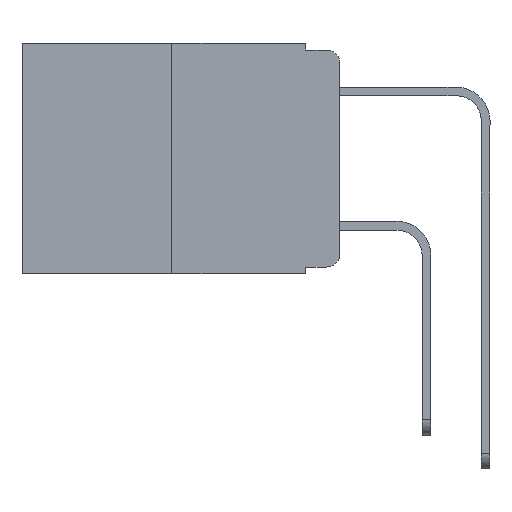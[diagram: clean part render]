
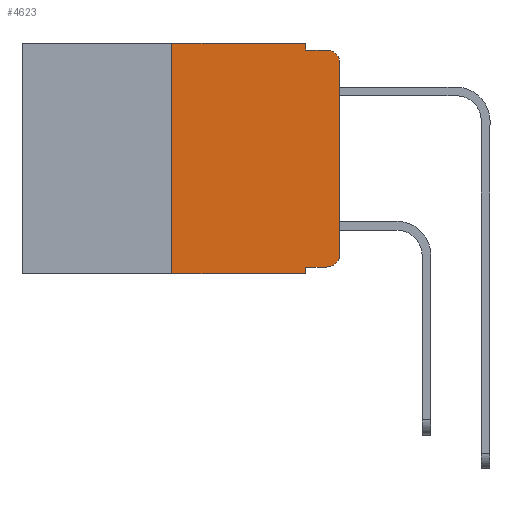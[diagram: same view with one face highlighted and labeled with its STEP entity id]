
A CAD part, left-side view. The second image highlights one B-rep face of the part: STEP entity #4623.
In plain terms, the highlighted planar face has unit normal (-1, 0, 0).
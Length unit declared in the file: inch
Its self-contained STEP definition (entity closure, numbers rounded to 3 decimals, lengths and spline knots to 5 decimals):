
#104 = VECTOR ( 'NONE', #4649, 39.37008 ) ;
#721 = ORIENTED_EDGE ( 'NONE', *, *, #9399, .F. ) ;
#742 = VERTEX_POINT ( 'NONE', #12933 ) ;
#1027 = AXIS2_PLACEMENT_3D ( 'NONE', #5376, #12724, #6508 ) ;
#1413 = CIRCLE ( 'NONE', #1027, 0.02 ) ;
#1497 = CARTESIAN_POINT ( 'NONE',  ( 0., 0.473, -0.343 ) ) ;
#1637 = DIRECTION ( 'NONE',  ( 0., -1., 0. ) ) ;
#1709 = CARTESIAN_POINT ( 'NONE',  ( 0., 0.02, -0.01 ) ) ;
#1729 = EDGE_LOOP ( 'NONE', ( #3747, #9186, #721, #8154, #5910, #5442, #3701, #11377, #7522, #10274 ) ) ;
#2589 = DIRECTION ( 'NONE',  ( 0., -1., 0. ) ) ;
#2990 = CARTESIAN_POINT ( 'NONE',  ( 0., 0.051, -0.333 ) ) ;
#2999 = LINE ( 'NONE', #11617, #8908 ) ;
#3168 = CARTESIAN_POINT ( 'NONE',  ( 0., 0.051, -0.343 ) ) ;
#3259 = VERTEX_POINT ( 'NONE', #11112 ) ;
#3571 = AXIS2_PLACEMENT_3D ( 'NONE', #6929, #10416, #8793 ) ;
#3701 = ORIENTED_EDGE ( 'NONE', *, *, #12202, .T. ) ;
#3729 = VERTEX_POINT ( 'NONE', #7700 ) ;
#3747 = ORIENTED_EDGE ( 'NONE', *, *, #4764, .T. ) ;
#3882 = CARTESIAN_POINT ( 'NONE',  ( 0., 0.473, 0. ) ) ;
#3914 = VECTOR ( 'NONE', #7093, 39.37008 ) ;
#4100 = EDGE_CURVE ( 'NONE', #3259, #742, #5727, .T. ) ;
#4226 = AXIS2_PLACEMENT_3D ( 'NONE', #11518, #11501, #5361 ) ;
#4256 = LINE ( 'NONE', #11847, #9707 ) ;
#4446 = VERTEX_POINT ( 'NONE', #7901 ) ;
#4544 = VERTEX_POINT ( 'NONE', #11835 ) ;
#4623 = ADVANCED_FACE ( 'NONE', ( #13670 ), #11587, .F. ) ;
#4649 = DIRECTION ( 'NONE',  ( 0., 0., -1. ) ) ;
#4717 = CARTESIAN_POINT ( 'NONE',  ( 0., 0.051, 0. ) ) ;
#4764 = EDGE_CURVE ( 'NONE', #4925, #4544, #12426, .T. ) ;
#4925 = VERTEX_POINT ( 'NONE', #12439 ) ;
#4958 = CIRCLE ( 'NONE', #3571, 0.02 ) ;
#5225 = DIRECTION ( 'NONE',  ( 0., 0., 1. ) ) ;
#5226 = DIRECTION ( 'NONE',  ( 0., 0., -1. ) ) ;
#5293 = LINE ( 'NONE', #7303, #8558 ) ;
#5361 = DIRECTION ( 'NONE',  ( 0., 0., -1. ) ) ;
#5376 = CARTESIAN_POINT ( 'NONE',  ( 0., 0.02, -0.313 ) ) ;
#5442 = ORIENTED_EDGE ( 'NONE', *, *, #9264, .F. ) ;
#5491 = VECTOR ( 'NONE', #1637, 39.37008 ) ;
#5637 = EDGE_CURVE ( 'NONE', #6915, #3729, #9873, .T. ) ;
#5727 = LINE ( 'NONE', #4717, #104 ) ;
#5807 = LINE ( 'NONE', #1497, #11384 ) ;
#5910 = ORIENTED_EDGE ( 'NONE', *, *, #9941, .F. ) ;
#5978 = VERTEX_POINT ( 'NONE', #1709 ) ;
#6288 = EDGE_CURVE ( 'NONE', #4544, #5978, #4958, .T. ) ;
#6392 = VERTEX_POINT ( 'NONE', #3168 ) ;
#6508 = DIRECTION ( 'NONE',  ( 0., 0., -1. ) ) ;
#6689 = EDGE_CURVE ( 'NONE', #6915, #6392, #5293, .T. ) ;
#6915 = VERTEX_POINT ( 'NONE', #2990 ) ;
#6929 = CARTESIAN_POINT ( 'NONE',  ( 0., 0.02, -0.03 ) ) ;
#6930 = CARTESIAN_POINT ( 'NONE',  ( 0., 0., 0. ) ) ;
#7093 = DIRECTION ( 'NONE',  ( 0., 0., 1. ) ) ;
#7303 = CARTESIAN_POINT ( 'NONE',  ( 0., 0.051, 0. ) ) ;
#7522 = ORIENTED_EDGE ( 'NONE', *, *, #5637, .T. ) ;
#7700 = CARTESIAN_POINT ( 'NONE',  ( 0., 0.02, -0.333 ) ) ;
#7901 = CARTESIAN_POINT ( 'NONE',  ( 0., 0.25, -0.343 ) ) ;
#8154 = ORIENTED_EDGE ( 'NONE', *, *, #4100, .F. ) ;
#8558 = VECTOR ( 'NONE', #5226, 39.37008 ) ;
#8793 = DIRECTION ( 'NONE',  ( 0., 0., -1. ) ) ;
#8813 = DIRECTION ( 'NONE',  ( 0., -1., 0. ) ) ;
#8828 = CARTESIAN_POINT ( 'NONE',  ( 0., 0.051, -0.333 ) ) ;
#8908 = VECTOR ( 'NONE', #5225, 39.37008 ) ;
#9186 = ORIENTED_EDGE ( 'NONE', *, *, #6288, .T. ) ;
#9264 = EDGE_CURVE ( 'NONE', #4446, #10966, #2999, .T. ) ;
#9399 = EDGE_CURVE ( 'NONE', #742, #5978, #4256, .T. ) ;
#9707 = VECTOR ( 'NONE', #13838, 39.37008 ) ;
#9873 = LINE ( 'NONE', #8828, #12265 ) ;
#9941 = EDGE_CURVE ( 'NONE', #10966, #3259, #11120, .T. ) ;
#10274 = ORIENTED_EDGE ( 'NONE', *, *, #11871, .T. ) ;
#10416 = DIRECTION ( 'NONE',  ( -1., 0., 0. ) ) ;
#10966 = VERTEX_POINT ( 'NONE', #12087 ) ;
#11112 = CARTESIAN_POINT ( 'NONE',  ( 0., 0.051, 0. ) ) ;
#11120 = LINE ( 'NONE', #3882, #5491 ) ;
#11377 = ORIENTED_EDGE ( 'NONE', *, *, #6689, .F. ) ;
#11384 = VECTOR ( 'NONE', #2589, 39.37008 ) ;
#11501 = DIRECTION ( 'NONE',  ( 1., 0., 0. ) ) ;
#11518 = CARTESIAN_POINT ( 'NONE',  ( 0., 0.473, 0. ) ) ;
#11587 = PLANE ( 'NONE',  #4226 ) ;
#11617 = CARTESIAN_POINT ( 'NONE',  ( 0., 0.25, 0. ) ) ;
#11835 = CARTESIAN_POINT ( 'NONE',  ( 0., 0., -0.03 ) ) ;
#11847 = CARTESIAN_POINT ( 'NONE',  ( 0., 0.051, -0.01 ) ) ;
#11871 = EDGE_CURVE ( 'NONE', #3729, #4925, #1413, .T. ) ;
#12087 = CARTESIAN_POINT ( 'NONE',  ( 0., 0.25, 0. ) ) ;
#12202 = EDGE_CURVE ( 'NONE', #4446, #6392, #5807, .T. ) ;
#12265 = VECTOR ( 'NONE', #8813, 39.37008 ) ;
#12426 = LINE ( 'NONE', #6930, #3914 ) ;
#12439 = CARTESIAN_POINT ( 'NONE',  ( 0., 0., -0.313 ) ) ;
#12724 = DIRECTION ( 'NONE',  ( -1., 0., 0. ) ) ;
#12933 = CARTESIAN_POINT ( 'NONE',  ( 0., 0.051, -0.01 ) ) ;
#13670 = FACE_OUTER_BOUND ( 'NONE', #1729, .T. ) ;
#13838 = DIRECTION ( 'NONE',  ( 0., -1., 0. ) ) ;
